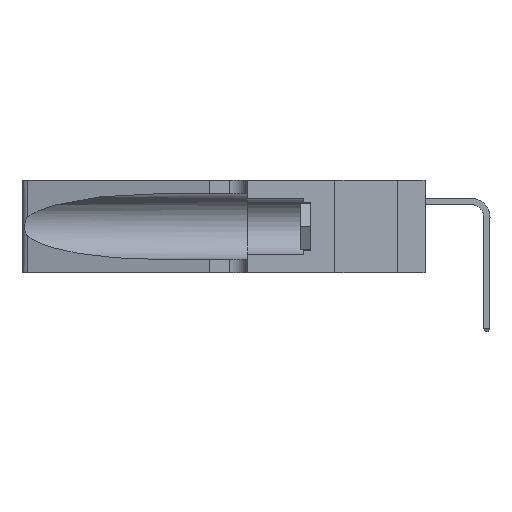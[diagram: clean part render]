
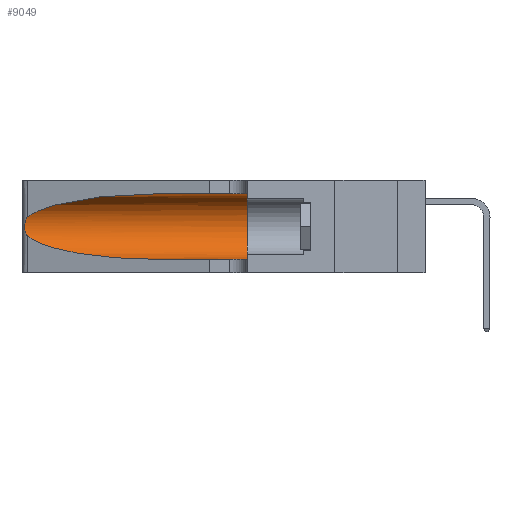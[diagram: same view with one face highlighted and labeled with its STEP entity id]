
A CAD part, left-side view. The second image highlights one B-rep face of the part: STEP entity #9049.
In plain terms, the highlighted cylindrical face has radius 3.308 mm (diameter 6.617 mm), a partial arc.
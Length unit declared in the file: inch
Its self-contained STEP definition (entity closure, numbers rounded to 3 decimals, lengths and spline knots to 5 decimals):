
#884 = ORIENTED_EDGE ( 'NONE', *, *, #23013, .F. ) ;
#975 = EDGE_CURVE ( 'NONE', #29009, #18174, #35083, .T. ) ;
#2436 = CARTESIAN_POINT ( 'NONE',  ( 0.26075, 1.23896, 0.178 ) ) ;
#2594 = VERTEX_POINT ( 'NONE', #18611 ) ;
#3341 = CARTESIAN_POINT ( 'NONE',  ( 0.1305, 1.61858, 0.31525 ) ) ;
#3484 = CARTESIAN_POINT ( 'NONE',  ( 0.25487, 1.22718, 0.14631 ) ) ;
#3567 = VECTOR ( 'NONE', #30133, 39.37008 ) ;
#5338 = CARTESIAN_POINT ( 'NONE',  ( 0.25487, 1.22718, 0.22369 ) ) ;
#5463 = CARTESIAN_POINT ( 'NONE',  ( 0.25856, 1.23593, 0.16098 ) ) ;
#7305 = ORIENTED_EDGE ( 'NONE', *, *, #32854, .T. ) ;
#7646 = VERTEX_POINT ( 'NONE', #22238 ) ;
#7859 = CARTESIAN_POINT ( 'NONE',  ( 0.25487, 1.22718, 0.14631 ) ) ;
#7995 = CARTESIAN_POINT ( 'NONE',  ( 0.1305, 0.35, 0.185 ) ) ;
#8530 = EDGE_LOOP ( 'NONE', ( #27539, #17660, #22155, #7305, #19493, #884 ) ) ;
#8565 = CARTESIAN_POINT ( 'NONE',  ( 0.25639, 1.23186, 0.15144 ) ) ;
#8716 = CARTESIAN_POINT ( 'NONE',  ( 0.2373, 1.15595, 0.28018 ) ) ;
#9049 = ADVANCED_FACE ( 'NONE', ( #22986 ), #22046, .F. ) ;
#10998 = LINE ( 'NONE', #28455, #25820 ) ;
#10999 = DIRECTION ( 'NONE',  ( 0., 0., 1. ) ) ;
#11582 = CARTESIAN_POINT ( 'NONE',  ( 0.25487, 1.22718, 0.14631 ) ) ;
#11743 = CARTESIAN_POINT ( 'NONE',  ( 0.25487, 1.22718, 0.22369 ) ) ;
#12345 = VERTEX_POINT ( 'NONE', #31816 ) ;
#12910 = EDGE_CURVE ( 'NONE', #2594, #12345, #26409, .T. ) ;
#13038 = AXIS2_PLACEMENT_3D ( 'NONE', #20890, #35369, #32570 ) ;
#13910 = CARTESIAN_POINT ( 'NONE',  ( 0.1305, 0.72297, 0.05475 ) ) ;
#14475 = CARTESIAN_POINT ( 'NONE',  ( 0.25639, 1.23184, 0.21858 ) ) ;
#16658 = AXIS2_PLACEMENT_3D ( 'NONE', #7995, #28714, #10999 ) ;
#17458 = CARTESIAN_POINT ( 'NONE',  ( 0.25854, 1.2359, 0.20912 ) ) ;
#17660 = ORIENTED_EDGE ( 'NONE', *, *, #36719, .T. ) ;
#18174 = VERTEX_POINT ( 'NONE', #23669 ) ;
#18611 = CARTESIAN_POINT ( 'NONE',  ( 0.1305, 0.35, 0.31525 ) ) ;
#19041 = VERTEX_POINT ( 'NONE', #3484 ) ;
#19493 = ORIENTED_EDGE ( 'NONE', *, *, #12910, .F. ) ;
#20387 = CARTESIAN_POINT ( 'NONE',  ( 0.26075, 1.23896, 0.19203 ) ) ;
#20459 = LINE ( 'NONE', #3341, #3567 ) ;
#20537 = CARTESIAN_POINT ( 'NONE',  ( 0.1305, 0.72297, 0.31525 ) ) ;
#20890 = CARTESIAN_POINT ( 'NONE',  ( 0.1305, 1.61858, 0.185 ) ) ;
#22046 = CYLINDRICAL_SURFACE ( 'NONE', #13038, 0.13025 ) ;
#22155 = ORIENTED_EDGE ( 'NONE', *, *, #37237, .T. ) ;
#22238 = CARTESIAN_POINT ( 'NONE',  ( 0.1305, 0.72297, 0.05475 ) ) ;
#22986 = FACE_OUTER_BOUND ( 'NONE', #8530, .T. ) ;
#23013 = EDGE_CURVE ( 'NONE', #29009, #2594, #20459, .T. ) ;
#23350 = CARTESIAN_POINT ( 'NONE',  ( 0.26017, 1.23833, 0.17102 ) ) ;
#23669 = CARTESIAN_POINT ( 'NONE',  ( 0.25487, 1.22718, 0.22369 ) ) ;
#25630 = CARTESIAN_POINT ( 'NONE',  ( 0.2373, 1.15595, 0.08982 ) ) ;
#25820 = VECTOR ( 'NONE', #31403, 39.37008 ) ;
#26176 = CARTESIAN_POINT ( 'NONE',  ( 0.25555, 1.22994, 0.2215 ) ) ;
#26304 = CARTESIAN_POINT ( 'NONE',  ( 0.25789, 1.23486, 0.15765 ) ) ;
#26409 = CIRCLE ( 'NONE', #16658, 0.13025 ) ;
#27539 = ORIENTED_EDGE ( 'NONE', *, *, #975, .T. ) ;
#28455 = CARTESIAN_POINT ( 'NONE',  ( 0.1305, 1.61858, 0.05475 ) ) ;
#28588 =( BOUNDED_CURVE ( )  B_SPLINE_CURVE ( 3, ( #7859, #25630, #31524, #13910 ),
 .UNSPECIFIED., .F., .T. ) 
 B_SPLINE_CURVE_WITH_KNOTS ( ( 4, 4 ),
 ( 3.44316, 4.71239 ),
 .UNSPECIFIED. ) 
 CURVE ( )  GEOMETRIC_REPRESENTATION_ITEM ( )  RATIONAL_B_SPLINE_CURVE ( ( 1., 0.87, 0.87, 1. ) ) 
 REPRESENTATION_ITEM ( '' )  );
#28714 = DIRECTION ( 'NONE',  ( 0., 1., 0. ) ) ;
#29009 = VERTEX_POINT ( 'NONE', #31331 ) ;
#29259 = CARTESIAN_POINT ( 'NONE',  ( 0.25555, 1.22993, 0.14849 ) ) ;
#29399 = CARTESIAN_POINT ( 'NONE',  ( 0.18966, 0.96281, 0.31525 ) ) ;
#30133 = DIRECTION ( 'NONE',  ( 0., -1., 0. ) ) ;
#31331 = CARTESIAN_POINT ( 'NONE',  ( 0.1305, 0.72297, 0.31525 ) ) ;
#31403 = DIRECTION ( 'NONE',  ( 0., -1., 0. ) ) ;
#31524 = CARTESIAN_POINT ( 'NONE',  ( 0.18966, 0.96281, 0.05475 ) ) ;
#31816 = CARTESIAN_POINT ( 'NONE',  ( 0.1305, 0.35, 0.05475 ) ) ;
#32570 = DIRECTION ( 'NONE',  ( 0., 0., -1. ) ) ;
#32854 = EDGE_CURVE ( 'NONE', #7646, #12345, #10998, .T. ) ;
#34984 = CARTESIAN_POINT ( 'NONE',  ( 0.25787, 1.23484, 0.2124 ) ) ;
#35083 =( BOUNDED_CURVE ( )  B_SPLINE_CURVE ( 3, ( #20537, #29399, #8716, #11743 ),
 .UNSPECIFIED., .F., .F. ) 
 B_SPLINE_CURVE_WITH_KNOTS ( ( 4, 4 ),
 ( 1.5708, 2.84003 ),
 .UNSPECIFIED. ) 
 CURVE ( )  GEOMETRIC_REPRESENTATION_ITEM ( )  RATIONAL_B_SPLINE_CURVE ( ( 1., 0.87, 0.87, 1. ) ) 
 REPRESENTATION_ITEM ( '' )  );
#35369 = DIRECTION ( 'NONE',  ( 0., -1., 0. ) ) ;
#35370 = B_SPLINE_CURVE_WITH_KNOTS ( 'NONE', 3,
 ( #5338, #26176, #14475, #34984, #17458, #37871, #20387, #2436, #23350, #5463, #26304, #8565, #29259, #11582 ),
 .UNSPECIFIED., .F., .F.,
 ( 4, 2, 2, 2, 2, 2, 4 ),
 ( 0., 0.00027, 0.00053, 0.00107, 0.0016, 0.00187, 0.00214 ),
 .UNSPECIFIED. ) ;
#36719 = EDGE_CURVE ( 'NONE', #18174, #19041, #35370, .T. ) ;
#37237 = EDGE_CURVE ( 'NONE', #19041, #7646, #28588, .T. ) ;
#37871 = CARTESIAN_POINT ( 'NONE',  ( 0.26018, 1.23835, 0.19895 ) ) ;
